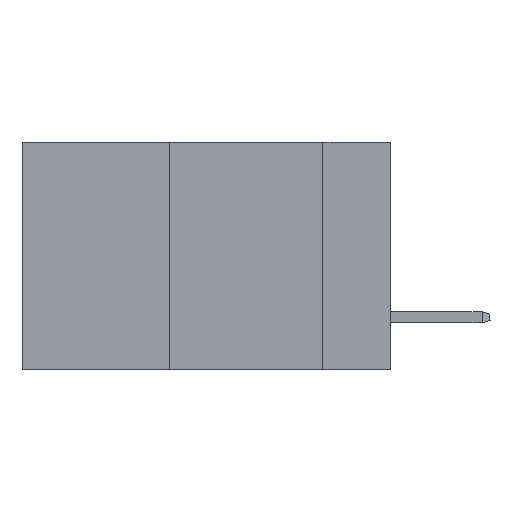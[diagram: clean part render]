
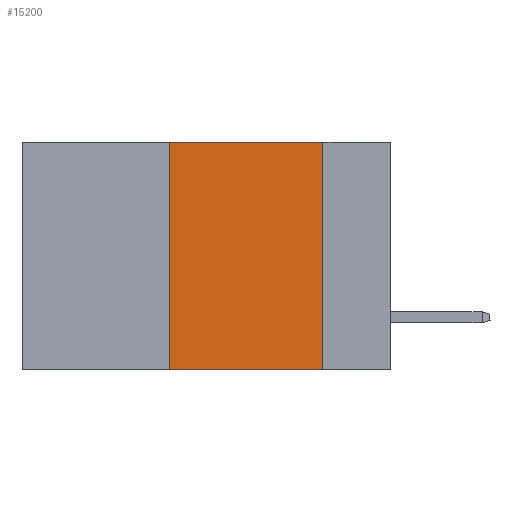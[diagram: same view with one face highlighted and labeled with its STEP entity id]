
A CAD part, left-side view. The second image highlights one B-rep face of the part: STEP entity #15200.
In plain terms, the highlighted planar face has unit normal (-1, 0, 0).
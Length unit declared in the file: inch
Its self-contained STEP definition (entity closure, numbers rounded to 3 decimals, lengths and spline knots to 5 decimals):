
#15 = ORIENTED_EDGE ( 'NONE', *, *, #17903, .T. ) ;
#364 = VERTEX_POINT ( 'NONE', #1975 ) ;
#647 = EDGE_LOOP ( 'NONE', ( #10087, #7129, #14188, #15 ) ) ;
#1261 = VECTOR ( 'NONE', #12539, 39.37008 ) ;
#1452 = VERTEX_POINT ( 'NONE', #6076 ) ;
#1538 = FACE_OUTER_BOUND ( 'NONE', #647, .T. ) ;
#1697 = DIRECTION ( 'NONE',  ( 1., 0., 0. ) ) ;
#1751 = LINE ( 'NONE', #2604, #1261 ) ;
#1975 = CARTESIAN_POINT ( 'NONE',  ( 0., 0.11, -0.37 ) ) ;
#2010 = EDGE_CURVE ( 'NONE', #1452, #12282, #6310, .T. ) ;
#2604 = CARTESIAN_POINT ( 'NONE',  ( 0., 0.36, 0. ) ) ;
#2657 = PLANE ( 'NONE',  #17427 ) ;
#3491 = CARTESIAN_POINT ( 'NONE',  ( 0., 0.6, 0. ) ) ;
#4669 = CARTESIAN_POINT ( 'NONE',  ( 0., 0.11, 0. ) ) ;
#5834 = DIRECTION ( 'NONE',  ( 0., -1., 0. ) ) ;
#6076 = CARTESIAN_POINT ( 'NONE',  ( 0., 0.36, 0. ) ) ;
#6077 = VERTEX_POINT ( 'NONE', #19447 ) ;
#6310 = LINE ( 'NONE', #19314, #13855 ) ;
#7129 = ORIENTED_EDGE ( 'NONE', *, *, #2010, .F. ) ;
#9856 = EDGE_CURVE ( 'NONE', #6077, #1452, #1751, .T. ) ;
#10087 = ORIENTED_EDGE ( 'NONE', *, *, #11268, .F. ) ;
#10489 = CARTESIAN_POINT ( 'NONE',  ( 0., 0.11, 0. ) ) ;
#11268 = EDGE_CURVE ( 'NONE', #12282, #364, #12750, .T. ) ;
#12282 = VERTEX_POINT ( 'NONE', #4669 ) ;
#12539 = DIRECTION ( 'NONE',  ( 0., 0., 1. ) ) ;
#12730 = LINE ( 'NONE', #16946, #19071 ) ;
#12750 = LINE ( 'NONE', #10489, #18380 ) ;
#13855 = VECTOR ( 'NONE', #5834, 39.37008 ) ;
#14188 = ORIENTED_EDGE ( 'NONE', *, *, #9856, .F. ) ;
#14838 = DIRECTION ( 'NONE',  ( 0., 0., -1. ) ) ;
#15200 = ADVANCED_FACE ( 'NONE', ( #1538 ), #2657, .F. ) ;
#16516 = DIRECTION ( 'NONE',  ( 0., 0., -1. ) ) ;
#16946 = CARTESIAN_POINT ( 'NONE',  ( 0., 0.6, -0.37 ) ) ;
#17143 = DIRECTION ( 'NONE',  ( 0., -1., 0. ) ) ;
#17427 = AXIS2_PLACEMENT_3D ( 'NONE', #3491, #1697, #14838 ) ;
#17903 = EDGE_CURVE ( 'NONE', #6077, #364, #12730, .T. ) ;
#18380 = VECTOR ( 'NONE', #16516, 39.37008 ) ;
#19071 = VECTOR ( 'NONE', #17143, 39.37008 ) ;
#19314 = CARTESIAN_POINT ( 'NONE',  ( 0., 0.6, 0. ) ) ;
#19447 = CARTESIAN_POINT ( 'NONE',  ( 0., 0.36, -0.37 ) ) ;
